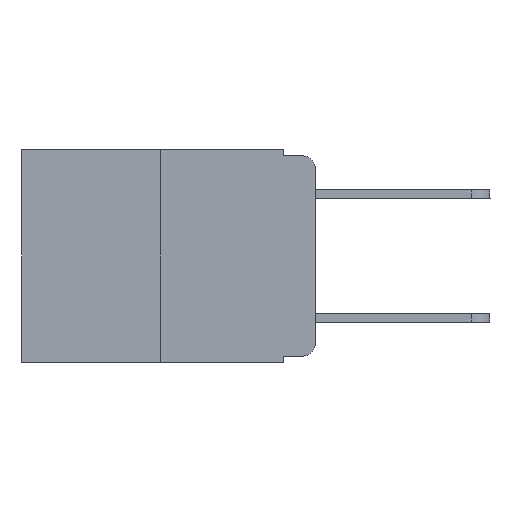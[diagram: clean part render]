
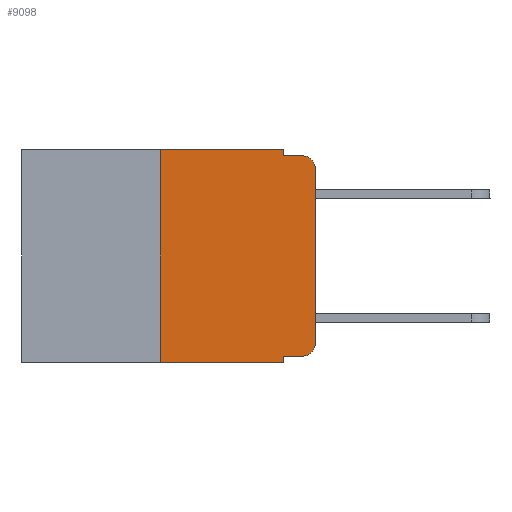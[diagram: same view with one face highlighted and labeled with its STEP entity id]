
A CAD part, left-side view. The second image highlights one B-rep face of the part: STEP entity #9098.
In plain terms, the highlighted planar face has unit normal (-1, 0, 0).
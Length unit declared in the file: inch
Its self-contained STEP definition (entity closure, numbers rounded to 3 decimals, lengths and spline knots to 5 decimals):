
#23 = LINE ( 'NONE', #10118, #10393 ) ;
#53 = DIRECTION ( 'NONE',  ( 0., -1., 0. ) ) ;
#88 = VERTEX_POINT ( 'NONE', #14782 ) ;
#118 = EDGE_CURVE ( 'NONE', #15736, #19590, #4800, .T. ) ;
#201 = DIRECTION ( 'NONE',  ( 1., 0., 0. ) ) ;
#711 = CIRCLE ( 'NONE', #15765, 0.02 ) ;
#992 = ORIENTED_EDGE ( 'NONE', *, *, #15249, .F. ) ;
#1125 = VECTOR ( 'NONE', #2804, 39.37008 ) ;
#1138 = CARTESIAN_POINT ( 'NONE',  ( 0., 0., -0.313 ) ) ;
#1498 = CARTESIAN_POINT ( 'NONE',  ( 0., 0.473, 0. ) ) ;
#1700 = LINE ( 'NONE', #14974, #7847 ) ;
#1796 = LINE ( 'NONE', #8513, #8347 ) ;
#1810 = CARTESIAN_POINT ( 'NONE',  ( 0., 0.02, -0.313 ) ) ;
#2215 = VERTEX_POINT ( 'NONE', #20662 ) ;
#2308 = ORIENTED_EDGE ( 'NONE', *, *, #9650, .T. ) ;
#2384 = CARTESIAN_POINT ( 'NONE',  ( 0., 0.25, -0.343 ) ) ;
#2769 = CARTESIAN_POINT ( 'NONE',  ( 0., 0.051, 0. ) ) ;
#2804 = DIRECTION ( 'NONE',  ( 0., 0., -1. ) ) ;
#2945 = DIRECTION ( 'NONE',  ( -1., 0., 0. ) ) ;
#3094 = CARTESIAN_POINT ( 'NONE',  ( 0., 0.02, -0.01 ) ) ;
#3375 = FACE_OUTER_BOUND ( 'NONE', #12842, .T. ) ;
#3462 = VERTEX_POINT ( 'NONE', #4976 ) ;
#4244 = EDGE_CURVE ( 'NONE', #10793, #3462, #1700, .T. ) ;
#4733 = EDGE_CURVE ( 'NONE', #11626, #19590, #16703, .T. ) ;
#4800 = CIRCLE ( 'NONE', #9026, 0.02 ) ;
#4856 = CARTESIAN_POINT ( 'NONE',  ( 0., 0.473, 0. ) ) ;
#4896 = DIRECTION ( 'NONE',  ( 0., -1., 0. ) ) ;
#4976 = CARTESIAN_POINT ( 'NONE',  ( 0., 0.051, -0.343 ) ) ;
#5117 = DIRECTION ( 'NONE',  ( -1., 0., 0. ) ) ;
#5454 = CARTESIAN_POINT ( 'NONE',  ( 0., 0., -0.03 ) ) ;
#6468 = EDGE_CURVE ( 'NONE', #13122, #88, #23, .T. ) ;
#6546 = PLANE ( 'NONE',  #10432 ) ;
#7442 = VECTOR ( 'NONE', #20467, 39.37008 ) ;
#7847 = VECTOR ( 'NONE', #4896, 39.37008 ) ;
#7850 = CARTESIAN_POINT ( 'NONE',  ( 0., 0.051, 0. ) ) ;
#7910 = DIRECTION ( 'NONE',  ( 0., 0., 1. ) ) ;
#8143 = DIRECTION ( 'NONE',  ( 0., -1., 0. ) ) ;
#8347 = VECTOR ( 'NONE', #21323, 39.37008 ) ;
#8513 = CARTESIAN_POINT ( 'NONE',  ( 0., 0., 0. ) ) ;
#8987 = CARTESIAN_POINT ( 'NONE',  ( 0., 0.051, -0.01 ) ) ;
#9026 = AXIS2_PLACEMENT_3D ( 'NONE', #19823, #2945, #16315 ) ;
#9098 = ADVANCED_FACE ( 'NONE', ( #3375 ), #6546, .F. ) ;
#9650 = EDGE_CURVE ( 'NONE', #13465, #15736, #1796, .T. ) ;
#9786 = ORIENTED_EDGE ( 'NONE', *, *, #19162, .T. ) ;
#10118 = CARTESIAN_POINT ( 'NONE',  ( 0., 0.051, -0.333 ) ) ;
#10393 = VECTOR ( 'NONE', #8143, 39.37008 ) ;
#10432 = AXIS2_PLACEMENT_3D ( 'NONE', #1498, #201, #11497 ) ;
#10485 = CARTESIAN_POINT ( 'NONE',  ( 0., 0.051, 0. ) ) ;
#10785 = DIRECTION ( 'NONE',  ( 0., 0., -1. ) ) ;
#10793 = VERTEX_POINT ( 'NONE', #2384 ) ;
#11225 = LINE ( 'NONE', #4856, #15860 ) ;
#11237 = ORIENTED_EDGE ( 'NONE', *, *, #118, .T. ) ;
#11497 = DIRECTION ( 'NONE',  ( 0., 0., -1. ) ) ;
#11533 = LINE ( 'NONE', #13392, #12391 ) ;
#11626 = VERTEX_POINT ( 'NONE', #8987 ) ;
#12391 = VECTOR ( 'NONE', #7910, 39.37008 ) ;
#12519 = ORIENTED_EDGE ( 'NONE', *, *, #16785, .F. ) ;
#12842 = EDGE_LOOP ( 'NONE', ( #2308, #11237, #16911, #19184, #992, #12519, #16344, #16895, #18638, #9786 ) ) ;
#13122 = VERTEX_POINT ( 'NONE', #18394 ) ;
#13392 = CARTESIAN_POINT ( 'NONE',  ( 0., 0.25, 0. ) ) ;
#13465 = VERTEX_POINT ( 'NONE', #1138 ) ;
#13784 = VECTOR ( 'NONE', #53, 39.37008 ) ;
#13925 = VERTEX_POINT ( 'NONE', #2769 ) ;
#14445 = EDGE_CURVE ( 'NONE', #13122, #3462, #20351, .T. ) ;
#14782 = CARTESIAN_POINT ( 'NONE',  ( 0., 0.02, -0.333 ) ) ;
#14974 = CARTESIAN_POINT ( 'NONE',  ( 0., 0.473, -0.343 ) ) ;
#15249 = EDGE_CURVE ( 'NONE', #2215, #13925, #11225, .T. ) ;
#15736 = VERTEX_POINT ( 'NONE', #5454 ) ;
#15765 = AXIS2_PLACEMENT_3D ( 'NONE', #1810, #5117, #10785 ) ;
#15769 = EDGE_CURVE ( 'NONE', #13925, #11626, #19461, .T. ) ;
#15860 = VECTOR ( 'NONE', #21301, 39.37008 ) ;
#16315 = DIRECTION ( 'NONE',  ( 0., 0., -1. ) ) ;
#16344 = ORIENTED_EDGE ( 'NONE', *, *, #4244, .T. ) ;
#16703 = LINE ( 'NONE', #18454, #13784 ) ;
#16785 = EDGE_CURVE ( 'NONE', #10793, #2215, #11533, .T. ) ;
#16895 = ORIENTED_EDGE ( 'NONE', *, *, #14445, .F. ) ;
#16911 = ORIENTED_EDGE ( 'NONE', *, *, #4733, .F. ) ;
#18394 = CARTESIAN_POINT ( 'NONE',  ( 0., 0.051, -0.333 ) ) ;
#18454 = CARTESIAN_POINT ( 'NONE',  ( 0., 0.051, -0.01 ) ) ;
#18638 = ORIENTED_EDGE ( 'NONE', *, *, #6468, .T. ) ;
#19162 = EDGE_CURVE ( 'NONE', #88, #13465, #711, .T. ) ;
#19184 = ORIENTED_EDGE ( 'NONE', *, *, #15769, .F. ) ;
#19461 = LINE ( 'NONE', #7850, #1125 ) ;
#19590 = VERTEX_POINT ( 'NONE', #3094 ) ;
#19823 = CARTESIAN_POINT ( 'NONE',  ( 0., 0.02, -0.03 ) ) ;
#20351 = LINE ( 'NONE', #10485, #7442 ) ;
#20467 = DIRECTION ( 'NONE',  ( 0., 0., -1. ) ) ;
#20662 = CARTESIAN_POINT ( 'NONE',  ( 0., 0.25, 0. ) ) ;
#21301 = DIRECTION ( 'NONE',  ( 0., -1., 0. ) ) ;
#21323 = DIRECTION ( 'NONE',  ( 0., 0., 1. ) ) ;
